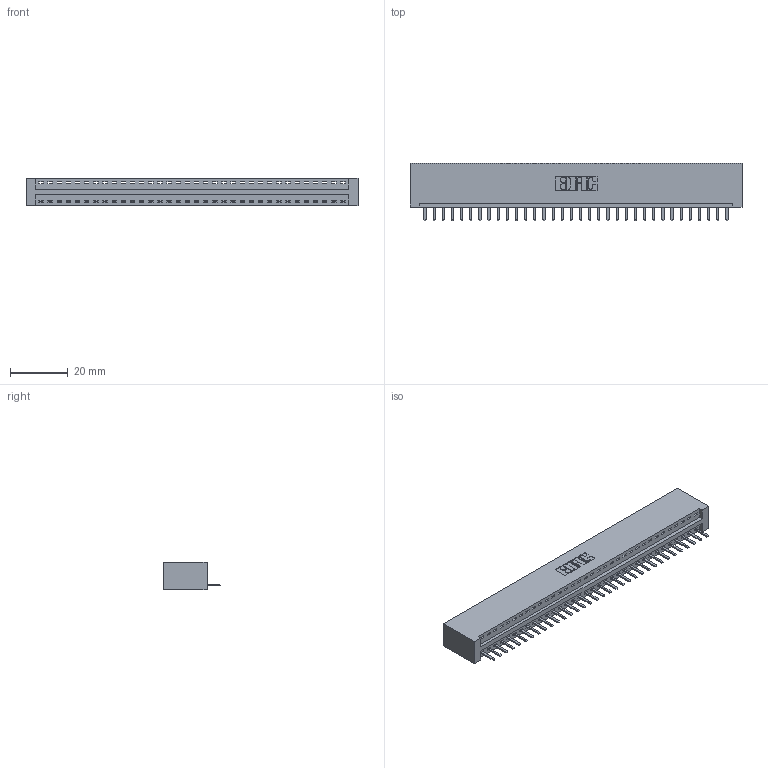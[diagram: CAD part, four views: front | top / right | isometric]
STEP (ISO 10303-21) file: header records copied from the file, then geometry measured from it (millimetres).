
FILE_DESCRIPTION (( 'STEP AP203' ), '1' );
FILE_NAME ('396-034-520-101.STEP', '2018-09-05T23:45:58', ( '' ), ( '' ), 'SwSTEP 2.0', 'SolidWorks 2016', '' );
FILE_SCHEMA (( 'CONFIG_CONTROL_DESIGN' ));
Length unit declared in the file: inch
Products named in the file (3): 345-292-001_345-293-120; 396-034-520-101; 346 Part_No Mounting Lugs
Assembly tree (35 placements, depth 2):
  396-034-520-101
    346 Part_No Mounting Lugs
    345-292-001_345-293-120  x34
Bounding box: 115.19 x 20.02 x 9.4 mm (x, y, z)
Volume: 11422.6 mm3; surface area: 13939.1 mm2
Topology: 35 solids, 35 shells, 2222 faces, 6561 edges, 4282 vertices
Faces by surface type: plane 1500, cylinder 722
Entity records: 22015 total; most frequent: CARTESIAN_POINT 3794, ORIENTED_EDGE 3750, DIRECTION 3339, EDGE_CURVE 1875, VECTOR 1611, LINE 1611, VERTEX_POINT 1246, AXIS2_PLACEMENT_3D 864
